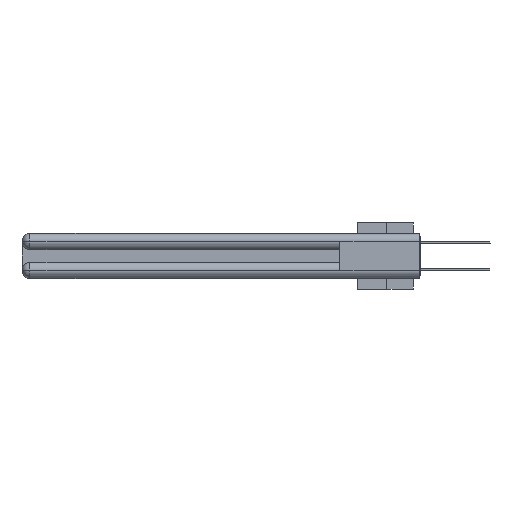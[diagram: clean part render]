
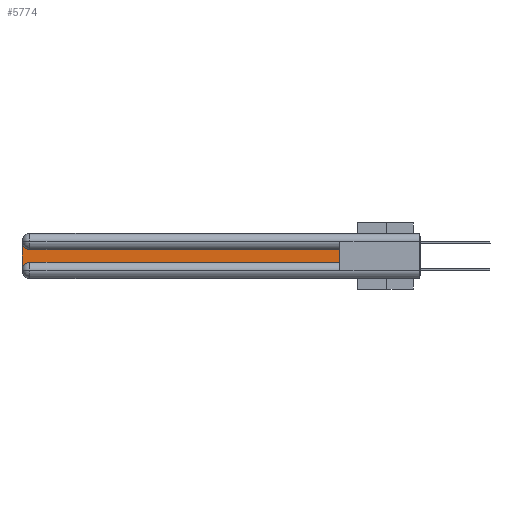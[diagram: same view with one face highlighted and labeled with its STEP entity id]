
A CAD part, left-side view. The second image highlights one B-rep face of the part: STEP entity #5774.
In plain terms, the highlighted planar face has unit normal (-1, 0, 0).
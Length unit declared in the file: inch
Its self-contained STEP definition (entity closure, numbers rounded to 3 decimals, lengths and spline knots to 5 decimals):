
#737 = ORIENTED_EDGE ( 'NONE', *, *, #3202, .T. ) ;
#746 = CARTESIAN_POINT ( 'NONE',  ( 0.075, 0.6, -0.2175 ) ) ;
#1039 = EDGE_CURVE ( 'NONE', #11154, #11078, #35258, .T. ) ;
#1086 = VERTEX_POINT ( 'NONE', #33814 ) ;
#1713 = VERTEX_POINT ( 'NONE', #29931 ) ;
#2112 = ORIENTED_EDGE ( 'NONE', *, *, #19143, .T. ) ;
#2887 = FACE_OUTER_BOUND ( 'NONE', #4037, .T. ) ;
#3202 = EDGE_CURVE ( 'NONE', #7183, #24987, #22623, .T. ) ;
#4021 = DIRECTION ( 'NONE',  ( 1., 0., 0. ) ) ;
#4037 = EDGE_LOOP ( 'NONE', ( #7251, #33240, #2112, #737, #8007, #26190 ) ) ;
#4385 = DIRECTION ( 'NONE',  ( 0., 0., -1. ) ) ;
#5774 = ADVANCED_FACE ( 'NONE', ( #2887 ), #20113, .F. ) ;
#5995 = VECTOR ( 'NONE', #13178, 39.37008 ) ;
#7183 = VERTEX_POINT ( 'NONE', #23172 ) ;
#7251 = ORIENTED_EDGE ( 'NONE', *, *, #10462, .T. ) ;
#7623 = CARTESIAN_POINT ( 'NONE',  ( 0.075, 0.6, -0.1225 ) ) ;
#7862 = DIRECTION ( 'NONE',  ( 1., 0., 0. ) ) ;
#8007 = ORIENTED_EDGE ( 'NONE', *, *, #15783, .T. ) ;
#8098 = CARTESIAN_POINT ( 'NONE',  ( 0.075, 2.94, -0.2175 ) ) ;
#8402 = VECTOR ( 'NONE', #14183, 39.37008 ) ;
#9052 = AXIS2_PLACEMENT_3D ( 'NONE', #33868, #20584, #22984 ) ;
#9494 = CARTESIAN_POINT ( 'NONE',  ( 0.075, 2.94, -0.2775 ) ) ;
#9829 = CARTESIAN_POINT ( 'NONE',  ( 0.075, 0.6, -0.2175 ) ) ;
#10462 = EDGE_CURVE ( 'NONE', #11078, #1713, #18409, .T. ) ;
#10672 = CARTESIAN_POINT ( 'NONE',  ( 0.075, 0.6, -0.1225 ) ) ;
#11078 = VERTEX_POINT ( 'NONE', #7623 ) ;
#11154 = VERTEX_POINT ( 'NONE', #29247 ) ;
#12039 = EDGE_CURVE ( 'NONE', #1713, #1086, #27785, .T. ) ;
#12569 = DIRECTION ( 'NONE',  ( 0., -1., 0. ) ) ;
#13178 = DIRECTION ( 'NONE',  ( 0., 1., 0. ) ) ;
#14183 = DIRECTION ( 'NONE',  ( 0., 0., -1. ) ) ;
#14808 = LINE ( 'NONE', #30575, #8402 ) ;
#14865 = LINE ( 'NONE', #9829, #34141 ) ;
#15488 = AXIS2_PLACEMENT_3D ( 'NONE', #21016, #7862, #29866 ) ;
#15783 = EDGE_CURVE ( 'NONE', #24987, #11154, #14865, .T. ) ;
#16845 = VECTOR ( 'NONE', #31065, 39.37008 ) ;
#18409 = LINE ( 'NONE', #10672, #5995 ) ;
#19143 = EDGE_CURVE ( 'NONE', #1086, #7183, #14808, .T. ) ;
#20113 = PLANE ( 'NONE',  #9052 ) ;
#20584 = DIRECTION ( 'NONE',  ( 1., 0., 0. ) ) ;
#21016 = CARTESIAN_POINT ( 'NONE',  ( 0.075, 2.94, -0.0625 ) ) ;
#22623 = CIRCLE ( 'NONE', #34892, 0.06 ) ;
#22984 = DIRECTION ( 'NONE',  ( 0., 0., -1. ) ) ;
#23172 = CARTESIAN_POINT ( 'NONE',  ( 0.075, 3., -0.2775 ) ) ;
#24987 = VERTEX_POINT ( 'NONE', #8098 ) ;
#26190 = ORIENTED_EDGE ( 'NONE', *, *, #1039, .T. ) ;
#27785 = CIRCLE ( 'NONE', #15488, 0.06 ) ;
#29247 = CARTESIAN_POINT ( 'NONE',  ( 0.075, 0.6, -0.2175 ) ) ;
#29866 = DIRECTION ( 'NONE',  ( 0., 0., -1. ) ) ;
#29931 = CARTESIAN_POINT ( 'NONE',  ( 0.075, 2.94, -0.1225 ) ) ;
#30575 = CARTESIAN_POINT ( 'NONE',  ( 0.075, 3., -0.2175 ) ) ;
#31065 = DIRECTION ( 'NONE',  ( 0., 0., 1. ) ) ;
#33240 = ORIENTED_EDGE ( 'NONE', *, *, #12039, .T. ) ;
#33814 = CARTESIAN_POINT ( 'NONE',  ( 0.075, 3., -0.0625 ) ) ;
#33868 = CARTESIAN_POINT ( 'NONE',  ( 0.075, 3., -0.1225 ) ) ;
#34141 = VECTOR ( 'NONE', #12569, 39.37008 ) ;
#34892 = AXIS2_PLACEMENT_3D ( 'NONE', #9494, #4021, #4385 ) ;
#35258 = LINE ( 'NONE', #746, #16845 ) ;
